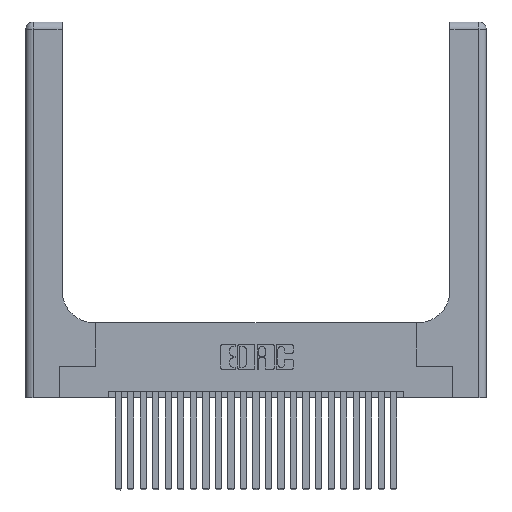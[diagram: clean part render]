
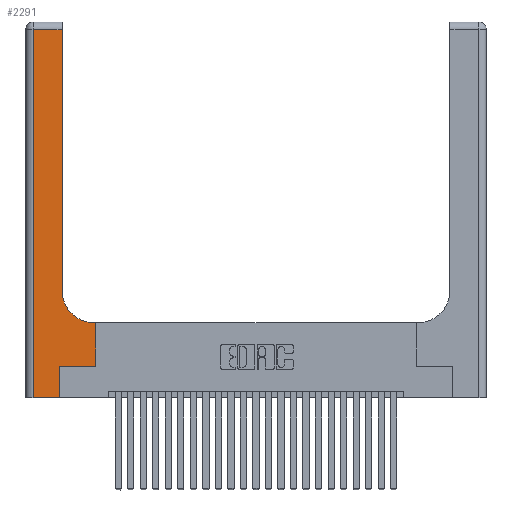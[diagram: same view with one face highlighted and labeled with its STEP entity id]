
A CAD part, top view. The second image highlights one B-rep face of the part: STEP entity #2291.
In plain terms, the highlighted planar face has unit normal (0, 0, 1).
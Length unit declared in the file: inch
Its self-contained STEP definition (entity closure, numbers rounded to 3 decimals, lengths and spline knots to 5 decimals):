
#1 = VERTEX_POINT ( 'NONE', #19361 ) ;
#66 = DIRECTION ( 'NONE',  ( 1., 0., 0. ) ) ;
#115 = CARTESIAN_POINT ( 'NONE',  ( 0.2915, 3., 0.37 ) ) ;
#171 = CARTESIAN_POINT ( 'NONE',  ( 0.5415, 0.85, 0.37 ) ) ;
#349 = DIRECTION ( 'NONE',  ( 0., -1., 0. ) ) ;
#1055 = VECTOR ( 'NONE', #66, 39.37008 ) ;
#1197 = VERTEX_POINT ( 'NONE', #24499 ) ;
#1642 = PLANE ( 'NONE',  #16538 ) ;
#2291 = ADVANCED_FACE ( 'NONE', ( #4490 ), #1642, .F. ) ;
#2899 = LINE ( 'NONE', #9778, #22074 ) ;
#3022 = EDGE_CURVE ( 'NONE', #23781, #22554, #2899, .T. ) ;
#3046 = CARTESIAN_POINT ( 'NONE',  ( 0.269, 0., 0.37 ) ) ;
#3074 = VECTOR ( 'NONE', #18698, 39.37008 ) ;
#3094 = EDGE_CURVE ( 'NONE', #25420, #10333, #24246, .T. ) ;
#3535 = LINE ( 'NONE', #115, #5689 ) ;
#3633 = CARTESIAN_POINT ( 'NONE',  ( 0., 3., 0.37 ) ) ;
#4408 = EDGE_CURVE ( 'NONE', #1, #19633, #8385, .T. ) ;
#4490 = FACE_OUTER_BOUND ( 'NONE', #15713, .T. ) ;
#4857 = CARTESIAN_POINT ( 'NONE',  ( 0.269, 0.25, 0.37 ) ) ;
#5364 = EDGE_CURVE ( 'NONE', #11171, #1197, #8345, .T. ) ;
#5445 = ORIENTED_EDGE ( 'NONE', *, *, #3022, .T. ) ;
#5447 = DIRECTION ( 'NONE',  ( 0., 0., -1. ) ) ;
#5689 = VECTOR ( 'NONE', #14034, 39.37008 ) ;
#5870 = CARTESIAN_POINT ( 'NONE',  ( 0.5585, 0.25, 0.37 ) ) ;
#5877 = AXIS2_PLACEMENT_3D ( 'NONE', #171, #15832, #21786 ) ;
#6116 = ORIENTED_EDGE ( 'NONE', *, *, #8781, .T. ) ;
#6372 = VECTOR ( 'NONE', #349, 39.37008 ) ;
#6965 = DIRECTION ( 'NONE',  ( -1., 0., 0. ) ) ;
#7634 = ORIENTED_EDGE ( 'NONE', *, *, #4408, .T. ) ;
#7788 = CARTESIAN_POINT ( 'NONE',  ( 0.06, 2.94, 0.37 ) ) ;
#8345 = LINE ( 'NONE', #18550, #14479 ) ;
#8385 = LINE ( 'NONE', #4857, #3074 ) ;
#8781 = EDGE_CURVE ( 'NONE', #23036, #23781, #3535, .T. ) ;
#9291 = DIRECTION ( 'NONE',  ( 0., 1., 0. ) ) ;
#9449 = DIRECTION ( 'NONE',  ( -1., 0., 0. ) ) ;
#9778 = CARTESIAN_POINT ( 'NONE',  ( 0., 2.94, 0.37 ) ) ;
#10333 = VERTEX_POINT ( 'NONE', #25205 ) ;
#10710 = ORIENTED_EDGE ( 'NONE', *, *, #5364, .T. ) ;
#11171 = VERTEX_POINT ( 'NONE', #20086 ) ;
#11914 = CARTESIAN_POINT ( 'NONE',  ( 0.06, 0., 0.37 ) ) ;
#12191 = CARTESIAN_POINT ( 'NONE',  ( 0.06, 3., 0.37 ) ) ;
#12821 = DIRECTION ( 'NONE',  ( 0., 1., 0. ) ) ;
#13017 = CARTESIAN_POINT ( 'NONE',  ( 0.2915, 0.85, 0.37 ) ) ;
#13844 = EDGE_CURVE ( 'NONE', #22554, #25420, #16902, .T. ) ;
#14034 = DIRECTION ( 'NONE',  ( 0., 1., 0. ) ) ;
#14175 = ORIENTED_EDGE ( 'NONE', *, *, #13844, .T. ) ;
#14479 = VECTOR ( 'NONE', #6965, 39.37008 ) ;
#15295 = ORIENTED_EDGE ( 'NONE', *, *, #3094, .T. ) ;
#15713 = EDGE_LOOP ( 'NONE', ( #6116, #5445, #14175, #15295, #17254, #7634, #23433, #10710, #16127 ) ) ;
#15832 = DIRECTION ( 'NONE',  ( 0., 0., -1. ) ) ;
#16127 = ORIENTED_EDGE ( 'NONE', *, *, #19046, .T. ) ;
#16386 = VECTOR ( 'NONE', #12821, 39.37008 ) ;
#16538 = AXIS2_PLACEMENT_3D ( 'NONE', #3633, #5447, #9449 ) ;
#16805 = LINE ( 'NONE', #3046, #19856 ) ;
#16902 = LINE ( 'NONE', #12191, #6372 ) ;
#17254 = ORIENTED_EDGE ( 'NONE', *, *, #21836, .T. ) ;
#17274 = CIRCLE ( 'NONE', #5877, 0.25 ) ;
#17389 = CARTESIAN_POINT ( 'NONE',  ( 0.2915, 2.94, 0.37 ) ) ;
#17897 = LINE ( 'NONE', #20692, #16386 ) ;
#18402 = EDGE_CURVE ( 'NONE', #19633, #11171, #17897, .T. ) ;
#18550 = CARTESIAN_POINT ( 'NONE',  ( 0.2915, 0.6, 0.37 ) ) ;
#18698 = DIRECTION ( 'NONE',  ( 1., 0., 0. ) ) ;
#19046 = EDGE_CURVE ( 'NONE', #1197, #23036, #17274, .T. ) ;
#19361 = CARTESIAN_POINT ( 'NONE',  ( 0.269, 0.25, 0.37 ) ) ;
#19633 = VERTEX_POINT ( 'NONE', #5870 ) ;
#19856 = VECTOR ( 'NONE', #9291, 39.37008 ) ;
#20086 = CARTESIAN_POINT ( 'NONE',  ( 0.5585, 0.6, 0.37 ) ) ;
#20692 = CARTESIAN_POINT ( 'NONE',  ( 0.5585, 0.25, 0.37 ) ) ;
#21762 = CARTESIAN_POINT ( 'NONE',  ( 0., 0., 0.37 ) ) ;
#21786 = DIRECTION ( 'NONE',  ( 1., 0., 0. ) ) ;
#21836 = EDGE_CURVE ( 'NONE', #10333, #1, #16805, .T. ) ;
#22074 = VECTOR ( 'NONE', #25423, 39.37008 ) ;
#22554 = VERTEX_POINT ( 'NONE', #7788 ) ;
#23036 = VERTEX_POINT ( 'NONE', #13017 ) ;
#23433 = ORIENTED_EDGE ( 'NONE', *, *, #18402, .T. ) ;
#23781 = VERTEX_POINT ( 'NONE', #17389 ) ;
#24246 = LINE ( 'NONE', #21762, #1055 ) ;
#24499 = CARTESIAN_POINT ( 'NONE',  ( 0.5415, 0.6, 0.37 ) ) ;
#25205 = CARTESIAN_POINT ( 'NONE',  ( 0.269, 0., 0.37 ) ) ;
#25420 = VERTEX_POINT ( 'NONE', #11914 ) ;
#25423 = DIRECTION ( 'NONE',  ( -1., 0., 0. ) ) ;
